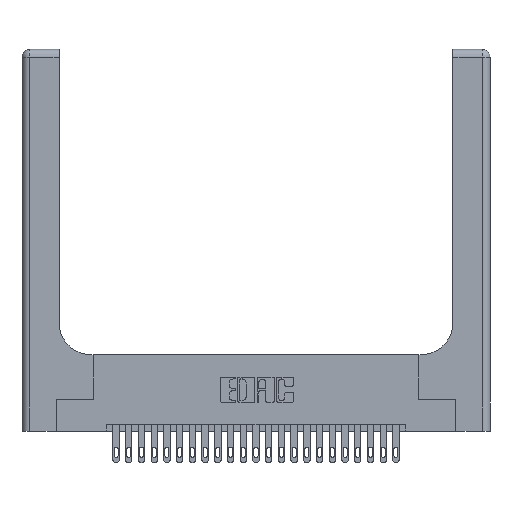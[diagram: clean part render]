
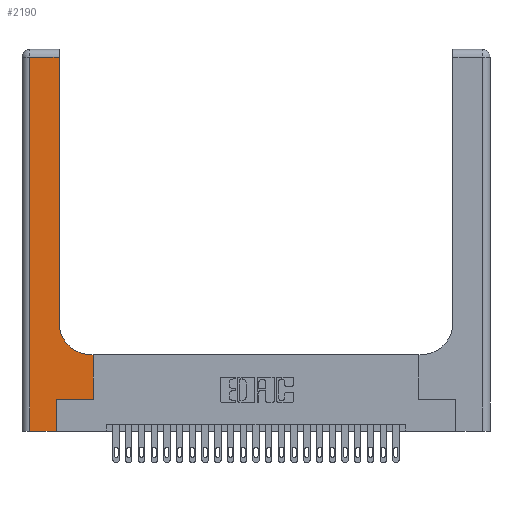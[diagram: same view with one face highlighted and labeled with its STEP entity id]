
A CAD part, top view. The second image highlights one B-rep face of the part: STEP entity #2190.
In plain terms, the highlighted planar face has unit normal (0, 0, 1).
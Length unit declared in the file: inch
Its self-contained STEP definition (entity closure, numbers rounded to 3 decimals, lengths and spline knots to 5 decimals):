
#552 = CARTESIAN_POINT ( 'NONE',  ( 0.5585, 0.25, 0.37 ) ) ;
#1023 = DIRECTION ( 'NONE',  ( 0., 1., 0. ) ) ;
#1340 = VECTOR ( 'NONE', #16186, 39.37008 ) ;
#1460 = VECTOR ( 'NONE', #1023, 39.37008 ) ;
#1541 = CARTESIAN_POINT ( 'NONE',  ( 0.269, 0.25, 0.37 ) ) ;
#1569 = ORIENTED_EDGE ( 'NONE', *, *, #10297, .T. ) ;
#1931 = VECTOR ( 'NONE', #16766, 39.37008 ) ;
#2190 = ADVANCED_FACE ( 'NONE', ( #20963 ), #19131, .F. ) ;
#2631 = CARTESIAN_POINT ( 'NONE',  ( 0.269, 0., 0.37 ) ) ;
#2645 = ORIENTED_EDGE ( 'NONE', *, *, #7615, .T. ) ;
#2827 = CARTESIAN_POINT ( 'NONE',  ( 0.269, 0., 0.37 ) ) ;
#2835 = ORIENTED_EDGE ( 'NONE', *, *, #7890, .T. ) ;
#2930 = EDGE_LOOP ( 'NONE', ( #23906, #17844, #2835, #12672, #2645, #6496, #1569, #24059, #22068 ) ) ;
#3040 = CARTESIAN_POINT ( 'NONE',  ( 0.5415, 0.85, 0.37 ) ) ;
#3639 = VERTEX_POINT ( 'NONE', #21299 ) ;
#3838 = LINE ( 'NONE', #12814, #1931 ) ;
#5057 = DIRECTION ( 'NONE',  ( 1., 0., 0. ) ) ;
#6144 = LINE ( 'NONE', #20769, #1460 ) ;
#6496 = ORIENTED_EDGE ( 'NONE', *, *, #10851, .T. ) ;
#6498 = VERTEX_POINT ( 'NONE', #24226 ) ;
#6642 = EDGE_CURVE ( 'NONE', #3639, #22751, #6144, .T. ) ;
#6713 = DIRECTION ( 'NONE',  ( 0., -1., 0. ) ) ;
#7615 = EDGE_CURVE ( 'NONE', #19300, #24829, #16951, .T. ) ;
#7812 = VERTEX_POINT ( 'NONE', #16718 ) ;
#7890 = EDGE_CURVE ( 'NONE', #23621, #7812, #22218, .T. ) ;
#8210 = DIRECTION ( 'NONE',  ( 0., 1., 0. ) ) ;
#8642 = EDGE_CURVE ( 'NONE', #22751, #23621, #10313, .T. ) ;
#9058 = EDGE_CURVE ( 'NONE', #7812, #19300, #3838, .T. ) ;
#10006 = VERTEX_POINT ( 'NONE', #22449 ) ;
#10297 = EDGE_CURVE ( 'NONE', #12786, #10006, #11823, .T. ) ;
#10313 = LINE ( 'NONE', #20299, #1340 ) ;
#10339 = VECTOR ( 'NONE', #6713, 39.37008 ) ;
#10851 = EDGE_CURVE ( 'NONE', #24829, #12786, #25547, .T. ) ;
#11823 = LINE ( 'NONE', #552, #15906 ) ;
#12672 = ORIENTED_EDGE ( 'NONE', *, *, #9058, .T. ) ;
#12786 = VERTEX_POINT ( 'NONE', #14636 ) ;
#12814 = CARTESIAN_POINT ( 'NONE',  ( 0., 0., 0.37 ) ) ;
#13384 = DIRECTION ( 'NONE',  ( 0., 1., 0. ) ) ;
#14636 = CARTESIAN_POINT ( 'NONE',  ( 0.5585, 0.25, 0.37 ) ) ;
#14864 = CARTESIAN_POINT ( 'NONE',  ( 0.06, 3., 0.37 ) ) ;
#15074 = EDGE_CURVE ( 'NONE', #6498, #3639, #24822, .T. ) ;
#15906 = VECTOR ( 'NONE', #8210, 39.37008 ) ;
#16186 = DIRECTION ( 'NONE',  ( -1., 0., 0. ) ) ;
#16569 = AXIS2_PLACEMENT_3D ( 'NONE', #23019, #21300, #21384 ) ;
#16718 = CARTESIAN_POINT ( 'NONE',  ( 0.06, 0., 0.37 ) ) ;
#16766 = DIRECTION ( 'NONE',  ( 1., 0., 0. ) ) ;
#16926 = DIRECTION ( 'NONE',  ( 0., 0., -1. ) ) ;
#16951 = LINE ( 'NONE', #2827, #25659 ) ;
#17081 = EDGE_CURVE ( 'NONE', #10006, #6498, #25672, .T. ) ;
#17286 = VECTOR ( 'NONE', #17879, 39.37008 ) ;
#17844 = ORIENTED_EDGE ( 'NONE', *, *, #8642, .T. ) ;
#17879 = DIRECTION ( 'NONE',  ( -1., 0., 0. ) ) ;
#17953 = CARTESIAN_POINT ( 'NONE',  ( 0.2915, 0.6, 0.37 ) ) ;
#18330 = CARTESIAN_POINT ( 'NONE',  ( 0.269, 0.25, 0.37 ) ) ;
#19131 = PLANE ( 'NONE',  #16569 ) ;
#19300 = VERTEX_POINT ( 'NONE', #2631 ) ;
#19334 = AXIS2_PLACEMENT_3D ( 'NONE', #3040, #16926, #5057 ) ;
#19487 = DIRECTION ( 'NONE',  ( 1., 0., 0. ) ) ;
#20299 = CARTESIAN_POINT ( 'NONE',  ( 0., 2.94, 0.37 ) ) ;
#20769 = CARTESIAN_POINT ( 'NONE',  ( 0.2915, 3., 0.37 ) ) ;
#20902 = CARTESIAN_POINT ( 'NONE',  ( 0.06, 2.94, 0.37 ) ) ;
#20963 = FACE_OUTER_BOUND ( 'NONE', #2930, .T. ) ;
#21299 = CARTESIAN_POINT ( 'NONE',  ( 0.2915, 0.85, 0.37 ) ) ;
#21300 = DIRECTION ( 'NONE',  ( 0., 0., -1. ) ) ;
#21384 = DIRECTION ( 'NONE',  ( -1., 0., 0. ) ) ;
#21884 = CARTESIAN_POINT ( 'NONE',  ( 0.2915, 2.94, 0.37 ) ) ;
#22068 = ORIENTED_EDGE ( 'NONE', *, *, #15074, .T. ) ;
#22218 = LINE ( 'NONE', #14864, #10339 ) ;
#22449 = CARTESIAN_POINT ( 'NONE',  ( 0.5585, 0.6, 0.37 ) ) ;
#22751 = VERTEX_POINT ( 'NONE', #21884 ) ;
#23019 = CARTESIAN_POINT ( 'NONE',  ( 0., 3., 0.37 ) ) ;
#23621 = VERTEX_POINT ( 'NONE', #20902 ) ;
#23906 = ORIENTED_EDGE ( 'NONE', *, *, #6642, .T. ) ;
#23965 = VECTOR ( 'NONE', #19487, 39.37008 ) ;
#24059 = ORIENTED_EDGE ( 'NONE', *, *, #17081, .T. ) ;
#24226 = CARTESIAN_POINT ( 'NONE',  ( 0.5415, 0.6, 0.37 ) ) ;
#24822 = CIRCLE ( 'NONE', #19334, 0.25 ) ;
#24829 = VERTEX_POINT ( 'NONE', #18330 ) ;
#25547 = LINE ( 'NONE', #1541, #23965 ) ;
#25659 = VECTOR ( 'NONE', #13384, 39.37008 ) ;
#25672 = LINE ( 'NONE', #17953, #17286 ) ;
